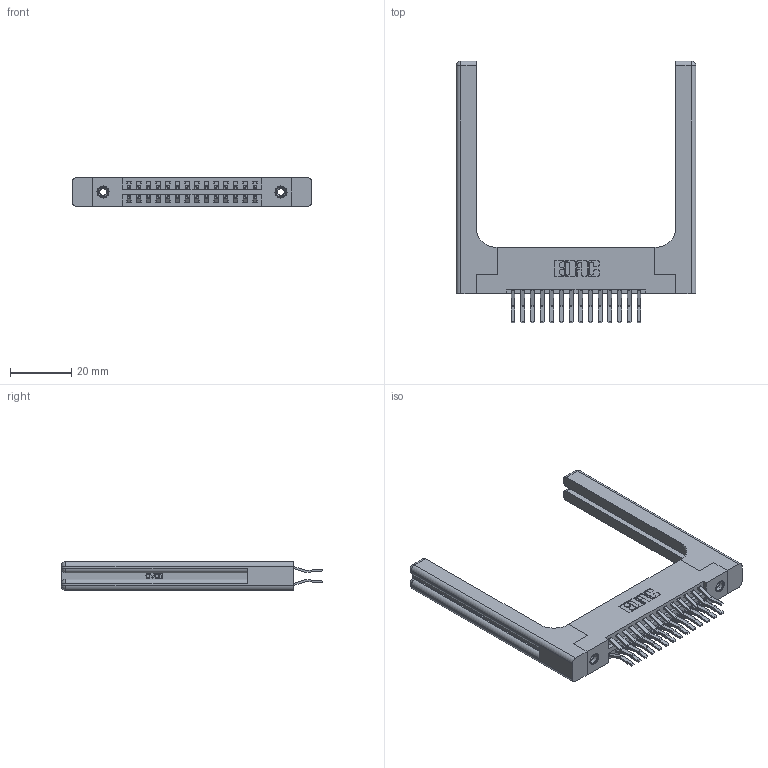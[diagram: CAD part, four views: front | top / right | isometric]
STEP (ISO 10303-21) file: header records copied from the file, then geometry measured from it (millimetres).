
FILE_DESCRIPTION (( 'STEP AP203' ), '1' );
FILE_NAME ('346-028-560-258.STEP', '2022-05-19T15:47:31', ( '' ), ( '' ), 'SwSTEP 2.0', 'SolidWorks 2020', '' );
FILE_SCHEMA (( 'CONFIG_CONTROL_DESIGN' ));
Length unit declared in the file: inch
Products named in the file (5): 345-292-001_560 Tail; 346 Part_Flush Mounting Lugs - 0.156 Dia-TH; 346-220-058_345-220-058; 346-028-560-258; 345-250-001_345-250-001-102
Assembly tree (33 placements, depth 2):
  346-028-560-258
    346 Part_Flush Mounting Lugs - 0.156 Dia-TH
    345-292-001_560 Tail  x28
    345-250-001_345-250-001-102  x2
    346-220-058_345-220-058  x2
Bounding box: 78.51 x 85.74 x 9.4 mm (x, y, z)
Volume: 15098 mm3; surface area: 15508.8 mm2
Topology: 33 solids, 33 shells, 1904 faces, 5539 edges, 3634 vertices
Faces by surface type: plane 1218, cylinder 626, bspline 36, cone 12, sphere 8, torus 4
Entity records: 18592 total; most frequent: CARTESIAN_POINT 4115, ORIENTED_EDGE 2844, DIRECTION 2614, EDGE_CURVE 1422, LINE 1138, VECTOR 1138, VERTEX_POINT 938, AXIS2_PLACEMENT_3D 738
